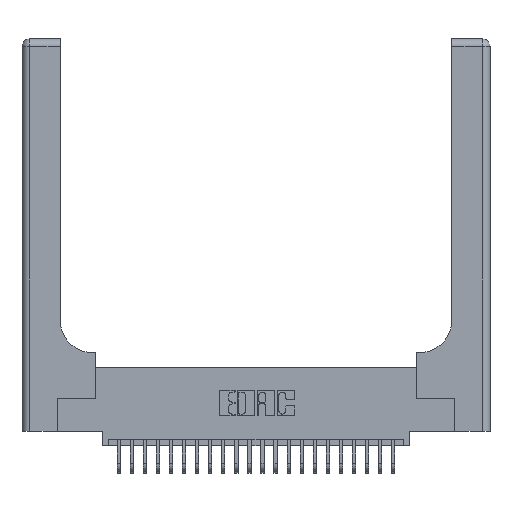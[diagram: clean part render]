
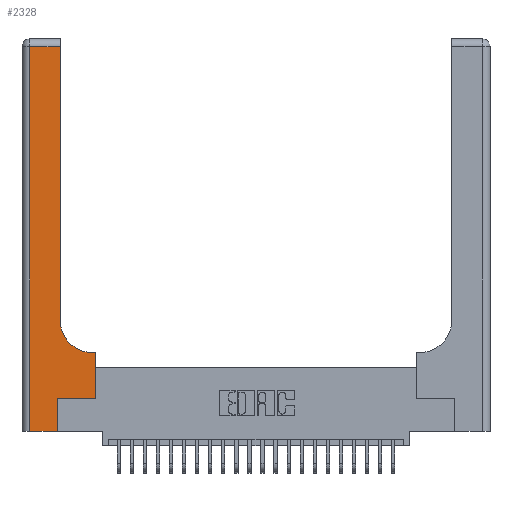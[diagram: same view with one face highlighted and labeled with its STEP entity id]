
A CAD part, top view. The second image highlights one B-rep face of the part: STEP entity #2328.
In plain terms, the highlighted planar face has unit normal (0, 0, 1).
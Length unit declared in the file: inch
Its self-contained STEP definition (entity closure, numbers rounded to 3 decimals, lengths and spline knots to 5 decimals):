
#76 = CARTESIAN_POINT ( 'NONE',  ( 0.2915, 3., 0.37 ) ) ;
#78 = LINE ( 'NONE', #2453, #4939 ) ;
#95 = EDGE_LOOP ( 'NONE', ( #26874, #8415, #4894, #17815, #1643, #19476, #19613, #5721, #18950 ) ) ;
#170 = LINE ( 'NONE', #25874, #15393 ) ;
#1643 = ORIENTED_EDGE ( 'NONE', *, *, #21348, .T. ) ;
#1829 = DIRECTION ( 'NONE',  ( -1., 0., 0. ) ) ;
#1897 = AXIS2_PLACEMENT_3D ( 'NONE', #9505, #24066, #13387 ) ;
#2157 = DIRECTION ( 'NONE',  ( 0., 1., 0. ) ) ;
#2328 = ADVANCED_FACE ( 'NONE', ( #17739 ), #10865, .F. ) ;
#2453 = CARTESIAN_POINT ( 'NONE',  ( 0.269, 0., 0.37 ) ) ;
#2626 = VERTEX_POINT ( 'NONE', #22660 ) ;
#2696 = EDGE_CURVE ( 'NONE', #9303, #2626, #12191, .T. ) ;
#3158 = VERTEX_POINT ( 'NONE', #23296 ) ;
#4656 = DIRECTION ( 'NONE',  ( 0., 0., -1. ) ) ;
#4894 = ORIENTED_EDGE ( 'NONE', *, *, #18343, .T. ) ;
#4939 = VECTOR ( 'NONE', #16702, 39.37008 ) ;
#5313 = EDGE_CURVE ( 'NONE', #20521, #9836, #12062, .T. ) ;
#5721 = ORIENTED_EDGE ( 'NONE', *, *, #2696, .T. ) ;
#5881 = CARTESIAN_POINT ( 'NONE',  ( 0.06, 2.94, 0.37 ) ) ;
#6102 = VERTEX_POINT ( 'NONE', #16531 ) ;
#8114 = EDGE_CURVE ( 'NONE', #9836, #20257, #170, .T. ) ;
#8176 = VECTOR ( 'NONE', #2157, 39.37008 ) ;
#8415 = ORIENTED_EDGE ( 'NONE', *, *, #8114, .T. ) ;
#8582 = VECTOR ( 'NONE', #16996, 39.37008 ) ;
#8819 = VERTEX_POINT ( 'NONE', #9930 ) ;
#8823 = DIRECTION ( 'NONE',  ( -1., 0., 0. ) ) ;
#9029 = CARTESIAN_POINT ( 'NONE',  ( 0.5585, 0.25, 0.37 ) ) ;
#9073 = EDGE_CURVE ( 'NONE', #23908, #8819, #14387, .T. ) ;
#9303 = VERTEX_POINT ( 'NONE', #22271 ) ;
#9505 = CARTESIAN_POINT ( 'NONE',  ( 0.5415, 0.85, 0.37 ) ) ;
#9836 = VERTEX_POINT ( 'NONE', #25716 ) ;
#9930 = CARTESIAN_POINT ( 'NONE',  ( 0.5585, 0.25, 0.37 ) ) ;
#10087 = LINE ( 'NONE', #23692, #26070 ) ;
#10742 = EDGE_CURVE ( 'NONE', #3158, #6102, #10087, .T. ) ;
#10865 = PLANE ( 'NONE',  #12122 ) ;
#12062 = LINE ( 'NONE', #76, #8176 ) ;
#12122 = AXIS2_PLACEMENT_3D ( 'NONE', #17047, #4656, #8823 ) ;
#12191 = LINE ( 'NONE', #18380, #17042 ) ;
#13329 = EDGE_CURVE ( 'NONE', #8819, #9303, #26934, .T. ) ;
#13387 = DIRECTION ( 'NONE',  ( 1., 0., 0. ) ) ;
#13587 = CARTESIAN_POINT ( 'NONE',  ( 0.269, 0.25, 0.37 ) ) ;
#14387 = LINE ( 'NONE', #13587, #8582 ) ;
#15147 = VECTOR ( 'NONE', #19275, 39.37008 ) ;
#15393 = VECTOR ( 'NONE', #1829, 39.37008 ) ;
#16364 = DIRECTION ( 'NONE',  ( -1., 0., 0. ) ) ;
#16531 = CARTESIAN_POINT ( 'NONE',  ( 0.269, 0., 0.37 ) ) ;
#16702 = DIRECTION ( 'NONE',  ( 0., 1., 0. ) ) ;
#16996 = DIRECTION ( 'NONE',  ( 1., 0., 0. ) ) ;
#17042 = VECTOR ( 'NONE', #16364, 39.37008 ) ;
#17047 = CARTESIAN_POINT ( 'NONE',  ( 0., 3., 0.37 ) ) ;
#17675 = DIRECTION ( 'NONE',  ( 1., 0., 0. ) ) ;
#17739 = FACE_OUTER_BOUND ( 'NONE', #95, .T. ) ;
#17815 = ORIENTED_EDGE ( 'NONE', *, *, #10742, .T. ) ;
#18343 = EDGE_CURVE ( 'NONE', #20257, #3158, #24656, .T. ) ;
#18380 = CARTESIAN_POINT ( 'NONE',  ( 0.2915, 0.6, 0.37 ) ) ;
#18950 = ORIENTED_EDGE ( 'NONE', *, *, #25107, .T. ) ;
#19064 = VECTOR ( 'NONE', #24078, 39.37008 ) ;
#19275 = DIRECTION ( 'NONE',  ( 0., 1., 0. ) ) ;
#19476 = ORIENTED_EDGE ( 'NONE', *, *, #9073, .T. ) ;
#19613 = ORIENTED_EDGE ( 'NONE', *, *, #13329, .T. ) ;
#20257 = VERTEX_POINT ( 'NONE', #5881 ) ;
#20521 = VERTEX_POINT ( 'NONE', #25745 ) ;
#21285 = CARTESIAN_POINT ( 'NONE',  ( 0.269, 0.25, 0.37 ) ) ;
#21348 = EDGE_CURVE ( 'NONE', #6102, #23908, #78, .T. ) ;
#21646 = CIRCLE ( 'NONE', #1897, 0.25 ) ;
#21958 = CARTESIAN_POINT ( 'NONE',  ( 0.06, 3., 0.37 ) ) ;
#22271 = CARTESIAN_POINT ( 'NONE',  ( 0.5585, 0.6, 0.37 ) ) ;
#22660 = CARTESIAN_POINT ( 'NONE',  ( 0.5415, 0.6, 0.37 ) ) ;
#23296 = CARTESIAN_POINT ( 'NONE',  ( 0.06, 0., 0.37 ) ) ;
#23692 = CARTESIAN_POINT ( 'NONE',  ( 0., 0., 0.37 ) ) ;
#23908 = VERTEX_POINT ( 'NONE', #21285 ) ;
#24066 = DIRECTION ( 'NONE',  ( 0., 0., -1. ) ) ;
#24078 = DIRECTION ( 'NONE',  ( 0., -1., 0. ) ) ;
#24656 = LINE ( 'NONE', #21958, #19064 ) ;
#25107 = EDGE_CURVE ( 'NONE', #2626, #20521, #21646, .T. ) ;
#25716 = CARTESIAN_POINT ( 'NONE',  ( 0.2915, 2.94, 0.37 ) ) ;
#25745 = CARTESIAN_POINT ( 'NONE',  ( 0.2915, 0.85, 0.37 ) ) ;
#25874 = CARTESIAN_POINT ( 'NONE',  ( 0., 2.94, 0.37 ) ) ;
#26070 = VECTOR ( 'NONE', #17675, 39.37008 ) ;
#26874 = ORIENTED_EDGE ( 'NONE', *, *, #5313, .T. ) ;
#26934 = LINE ( 'NONE', #9029, #15147 ) ;
